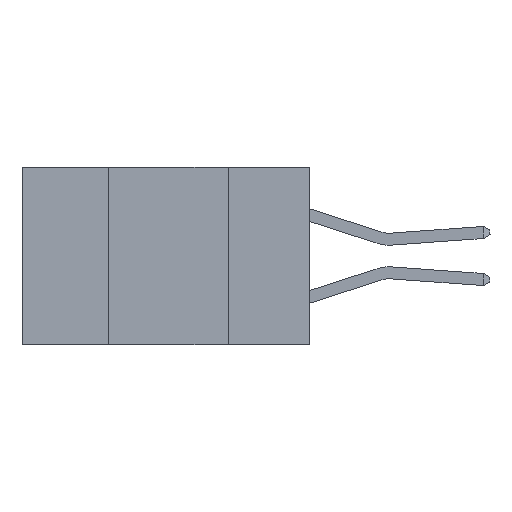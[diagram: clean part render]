
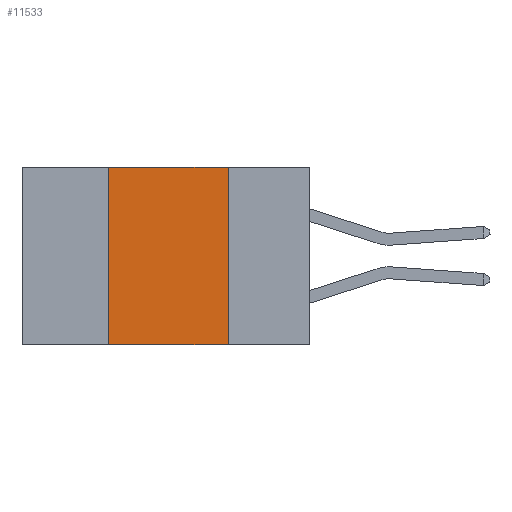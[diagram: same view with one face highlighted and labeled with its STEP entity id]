
A CAD part, left-side view. The second image highlights one B-rep face of the part: STEP entity #11533.
In plain terms, the highlighted planar face has unit normal (-1, 0, 0).
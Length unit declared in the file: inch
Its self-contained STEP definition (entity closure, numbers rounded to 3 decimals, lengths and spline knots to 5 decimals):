
#949 = DIRECTION ( 'NONE',  ( 0., 0., -1. ) ) ;
#1567 = LINE ( 'NONE', #6956, #3551 ) ;
#1962 = ORIENTED_EDGE ( 'NONE', *, *, #15250, .F. ) ;
#1976 = DIRECTION ( 'NONE',  ( 0., 0., -1. ) ) ;
#2020 = LINE ( 'NONE', #16672, #4980 ) ;
#2346 = CARTESIAN_POINT ( 'NONE',  ( 0., 0.17, -0.37 ) ) ;
#3192 = VERTEX_POINT ( 'NONE', #5986 ) ;
#3551 = VECTOR ( 'NONE', #4365, 39.37008 ) ;
#4365 = DIRECTION ( 'NONE',  ( 0., 0., 1. ) ) ;
#4424 = PLANE ( 'NONE',  #8861 ) ;
#4637 = DIRECTION ( 'NONE',  ( 0., -1., 0. ) ) ;
#4681 = VERTEX_POINT ( 'NONE', #5463 ) ;
#4980 = VECTOR ( 'NONE', #4637, 39.37008 ) ;
#5156 = VERTEX_POINT ( 'NONE', #13153 ) ;
#5323 = FACE_OUTER_BOUND ( 'NONE', #15321, .T. ) ;
#5463 = CARTESIAN_POINT ( 'NONE',  ( 0., 0.17, -0.37 ) ) ;
#5608 = VECTOR ( 'NONE', #16194, 39.37008 ) ;
#5986 = CARTESIAN_POINT ( 'NONE',  ( 0., 0.17, 0. ) ) ;
#6811 = ORIENTED_EDGE ( 'NONE', *, *, #9141, .F. ) ;
#6956 = CARTESIAN_POINT ( 'NONE',  ( 0., 0.42, -0.37 ) ) ;
#8861 = AXIS2_PLACEMENT_3D ( 'NONE', #9291, #10193, #1976 ) ;
#9141 = EDGE_CURVE ( 'NONE', #5156, #10267, #1567, .T. ) ;
#9291 = CARTESIAN_POINT ( 'NONE',  ( 0., 0.6, 0. ) ) ;
#10193 = DIRECTION ( 'NONE',  ( 1., 0., 0. ) ) ;
#10267 = VERTEX_POINT ( 'NONE', #15730 ) ;
#11140 = CARTESIAN_POINT ( 'NONE',  ( 0., 0.6, 0. ) ) ;
#11362 = EDGE_CURVE ( 'NONE', #3192, #4681, #14233, .T. ) ;
#11533 = ADVANCED_FACE ( 'NONE', ( #5323 ), #4424, .F. ) ;
#12361 = LINE ( 'NONE', #11140, #5608 ) ;
#12430 = EDGE_CURVE ( 'NONE', #5156, #4681, #2020, .T. ) ;
#12530 = ORIENTED_EDGE ( 'NONE', *, *, #11362, .F. ) ;
#13012 = VECTOR ( 'NONE', #949, 39.37008 ) ;
#13153 = CARTESIAN_POINT ( 'NONE',  ( 0., 0.42, -0.37 ) ) ;
#14233 = LINE ( 'NONE', #2346, #13012 ) ;
#15250 = EDGE_CURVE ( 'NONE', #10267, #3192, #12361, .T. ) ;
#15321 = EDGE_LOOP ( 'NONE', ( #12530, #1962, #6811, #15734 ) ) ;
#15730 = CARTESIAN_POINT ( 'NONE',  ( 0., 0.42, 0. ) ) ;
#15734 = ORIENTED_EDGE ( 'NONE', *, *, #12430, .T. ) ;
#16194 = DIRECTION ( 'NONE',  ( 0., -1., 0. ) ) ;
#16672 = CARTESIAN_POINT ( 'NONE',  ( 0., 0.6, -0.37 ) ) ;
